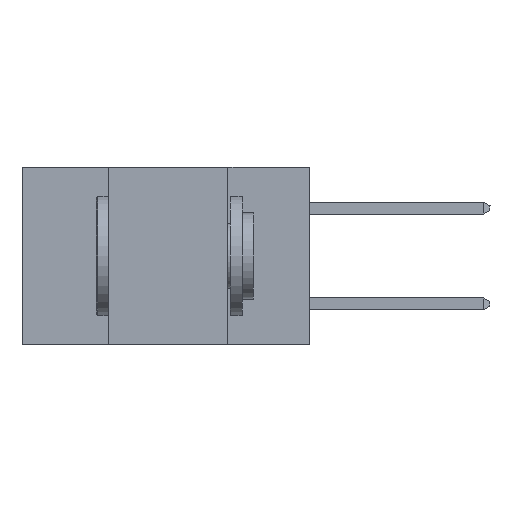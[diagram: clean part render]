
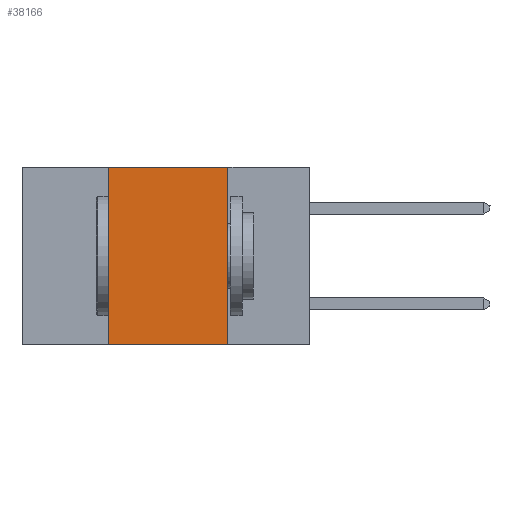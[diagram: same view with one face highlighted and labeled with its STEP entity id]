
A CAD part, left-side view. The second image highlights one B-rep face of the part: STEP entity #38166.
In plain terms, the highlighted planar face has unit normal (-1, 0, 0).
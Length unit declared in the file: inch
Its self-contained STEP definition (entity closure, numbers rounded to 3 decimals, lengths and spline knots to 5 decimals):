
#289 = CARTESIAN_POINT ( 'NONE',  ( 0., 0.17, 0. ) ) ;
#611 = EDGE_CURVE ( 'NONE', #35717, #22428, #5613, .T. ) ;
#4666 = EDGE_CURVE ( 'NONE', #22428, #26958, #25619, .T. ) ;
#5613 = LINE ( 'NONE', #40480, #15145 ) ;
#6544 = LINE ( 'NONE', #28333, #31406 ) ;
#7113 = ORIENTED_EDGE ( 'NONE', *, *, #16928, .F. ) ;
#7664 = VECTOR ( 'NONE', #37834, 39.37008 ) ;
#8755 = LINE ( 'NONE', #9776, #7664 ) ;
#9168 = CARTESIAN_POINT ( 'NONE',  ( 0., 0.17, -0.37 ) ) ;
#9776 = CARTESIAN_POINT ( 'NONE',  ( 0., 0.6, -0.37 ) ) ;
#11088 = DIRECTION ( 'NONE',  ( 0., 0., -1. ) ) ;
#12895 = CARTESIAN_POINT ( 'NONE',  ( 0., 0.42, -0.37 ) ) ;
#15145 = VECTOR ( 'NONE', #23149, 39.37008 ) ;
#16928 = EDGE_CURVE ( 'NONE', #34019, #35717, #6544, .T. ) ;
#17639 = PLANE ( 'NONE',  #33184 ) ;
#21168 = DIRECTION ( 'NONE',  ( 1., 0., 0. ) ) ;
#22428 = VERTEX_POINT ( 'NONE', #31058 ) ;
#23149 = DIRECTION ( 'NONE',  ( 0., -1., 0. ) ) ;
#24305 = ORIENTED_EDGE ( 'NONE', *, *, #4666, .F. ) ;
#24539 = VECTOR ( 'NONE', #11088, 39.37008 ) ;
#25619 = LINE ( 'NONE', #289, #24539 ) ;
#26958 = VERTEX_POINT ( 'NONE', #9168 ) ;
#28333 = CARTESIAN_POINT ( 'NONE',  ( 0., 0.42, 0. ) ) ;
#31058 = CARTESIAN_POINT ( 'NONE',  ( 0., 0.17, 0. ) ) ;
#31406 = VECTOR ( 'NONE', #38745, 39.37008 ) ;
#31413 = ORIENTED_EDGE ( 'NONE', *, *, #611, .F. ) ;
#31592 = CARTESIAN_POINT ( 'NONE',  ( 0., 0.6, 0. ) ) ;
#33184 = AXIS2_PLACEMENT_3D ( 'NONE', #31592, #21168, #45432 ) ;
#34019 = VERTEX_POINT ( 'NONE', #12895 ) ;
#34681 = EDGE_LOOP ( 'NONE', ( #24305, #31413, #7113, #40004 ) ) ;
#35717 = VERTEX_POINT ( 'NONE', #36612 ) ;
#36612 = CARTESIAN_POINT ( 'NONE',  ( 0., 0.42, 0. ) ) ;
#37834 = DIRECTION ( 'NONE',  ( 0., -1., 0. ) ) ;
#38166 = ADVANCED_FACE ( 'NONE', ( #42889 ), #17639, .F. ) ;
#38745 = DIRECTION ( 'NONE',  ( 0., 0., 1. ) ) ;
#40004 = ORIENTED_EDGE ( 'NONE', *, *, #44294, .T. ) ;
#40480 = CARTESIAN_POINT ( 'NONE',  ( 0., 0.6, 0. ) ) ;
#42889 = FACE_OUTER_BOUND ( 'NONE', #34681, .T. ) ;
#44294 = EDGE_CURVE ( 'NONE', #34019, #26958, #8755, .T. ) ;
#45432 = DIRECTION ( 'NONE',  ( 0., 0., -1. ) ) ;
